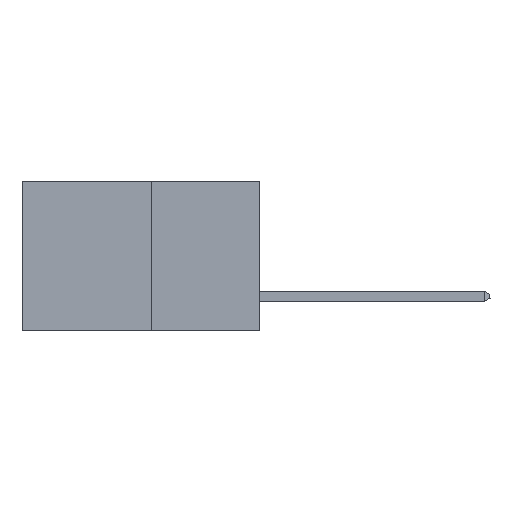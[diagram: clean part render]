
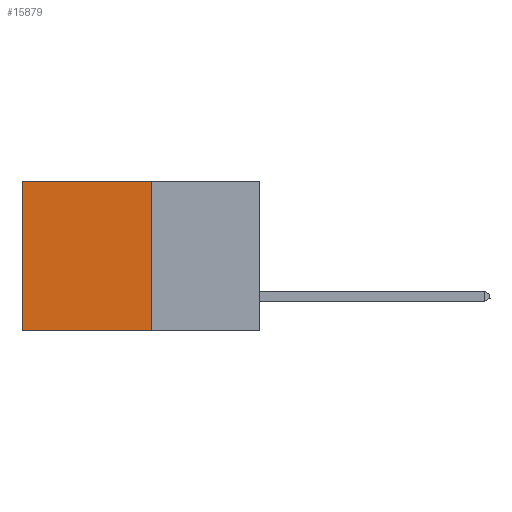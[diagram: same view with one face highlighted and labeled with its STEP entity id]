
A CAD part, left-side view. The second image highlights one B-rep face of the part: STEP entity #15879.
In plain terms, the highlighted planar face has unit normal (-1, 0, 0).
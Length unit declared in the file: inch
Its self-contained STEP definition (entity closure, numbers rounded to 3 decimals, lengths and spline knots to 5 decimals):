
#5 = CARTESIAN_POINT ( 'NONE',  ( 0.277, 0.27, 0. ) ) ;
#359 = CARTESIAN_POINT ( 'NONE',  ( 0.277, 0.27, -0.37 ) ) ;
#1416 = ORIENTED_EDGE ( 'NONE', *, *, #18822, .T. ) ;
#2346 = VERTEX_POINT ( 'NONE', #11003 ) ;
#4016 = LINE ( 'NONE', #359, #17702 ) ;
#4178 = EDGE_CURVE ( 'NONE', #14376, #2346, #23614, .T. ) ;
#4851 = LINE ( 'NONE', #5, #17020 ) ;
#5017 = DIRECTION ( 'NONE',  ( 0., 0., -1. ) ) ;
#5441 = CARTESIAN_POINT ( 'NONE',  ( 0.277, 0.27, -0.37 ) ) ;
#6611 = AXIS2_PLACEMENT_3D ( 'NONE', #5441, #24965, #10290 ) ;
#7020 = VERTEX_POINT ( 'NONE', #23036 ) ;
#9127 = FACE_OUTER_BOUND ( 'NONE', #18161, .T. ) ;
#10290 = DIRECTION ( 'NONE',  ( 0., 0., -1. ) ) ;
#11003 = CARTESIAN_POINT ( 'NONE',  ( 0.277, 0.59, -0.37 ) ) ;
#11351 = VECTOR ( 'NONE', #30533, 39.37008 ) ;
#14376 = VERTEX_POINT ( 'NONE', #27845 ) ;
#14423 = ORIENTED_EDGE ( 'NONE', *, *, #4178, .F. ) ;
#15879 = ADVANCED_FACE ( 'NONE', ( #9127 ), #20067, .F. ) ;
#16214 = EDGE_CURVE ( 'NONE', #7020, #2346, #25951, .T. ) ;
#16275 = DIRECTION ( 'NONE',  ( 0., 0., -1. ) ) ;
#16886 = DIRECTION ( 'NONE',  ( 0., 1., 0. ) ) ;
#17020 = VECTOR ( 'NONE', #16886, 39.37008 ) ;
#17702 = VECTOR ( 'NONE', #5017, 39.37008 ) ;
#18161 = EDGE_LOOP ( 'NONE', ( #24573, #14423, #24740, #1416 ) ) ;
#18822 = EDGE_CURVE ( 'NONE', #23353, #7020, #4851, .T. ) ;
#20067 = PLANE ( 'NONE',  #6611 ) ;
#20158 = EDGE_CURVE ( 'NONE', #23353, #14376, #4016, .T. ) ;
#23036 = CARTESIAN_POINT ( 'NONE',  ( 0.277, 0.59, 0. ) ) ;
#23353 = VERTEX_POINT ( 'NONE', #31314 ) ;
#23614 = LINE ( 'NONE', #30006, #11351 ) ;
#23652 = CARTESIAN_POINT ( 'NONE',  ( 0.277, 0.59, -0.37 ) ) ;
#24573 = ORIENTED_EDGE ( 'NONE', *, *, #16214, .T. ) ;
#24740 = ORIENTED_EDGE ( 'NONE', *, *, #20158, .F. ) ;
#24965 = DIRECTION ( 'NONE',  ( 1., 0., 0. ) ) ;
#25951 = LINE ( 'NONE', #23652, #30837 ) ;
#27845 = CARTESIAN_POINT ( 'NONE',  ( 0.277, 0.27, -0.37 ) ) ;
#30006 = CARTESIAN_POINT ( 'NONE',  ( 0.277, 0.27, -0.37 ) ) ;
#30533 = DIRECTION ( 'NONE',  ( 0., 1., 0. ) ) ;
#30837 = VECTOR ( 'NONE', #16275, 39.37008 ) ;
#31314 = CARTESIAN_POINT ( 'NONE',  ( 0.277, 0.27, 0. ) ) ;
